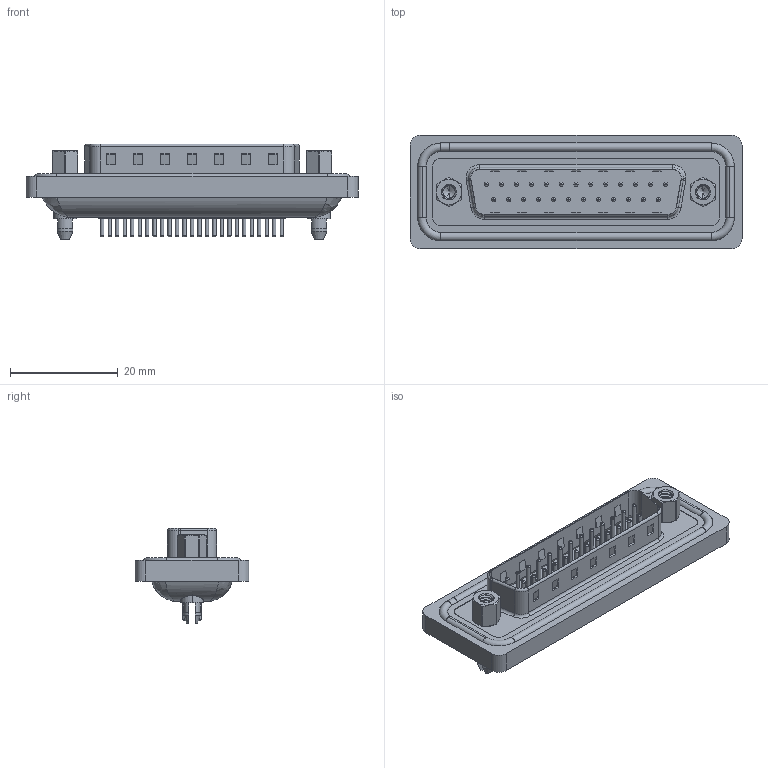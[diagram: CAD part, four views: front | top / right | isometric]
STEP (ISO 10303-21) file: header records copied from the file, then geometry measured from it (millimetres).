
FILE_DESCRIPTION (( 'STEP AP203' ), '1' );
FILE_NAME ('627-W25-220-013.STEP', '2021-04-05T19:34:12', ( '' ), ( '' ), 'SwSTEP 2.0', 'SolidWorks 2020', '' );
FILE_SCHEMA (( 'CONFIG_CONTROL_DESIGN' ));
Length unit declared in the file: millimetre
Products named in the file (8): 627W Contact Row 1_20; 627-W25-220-013; 627W Contact Row 2_20; 627W Shell Front_25 Contacts; 627W 4-40 Hex Standoff; 627W Waterproof Housing_25 Contacts BL; 627W Housing_25 Contacts; 627W 4-40 Threaded Boardlock
Assembly tree (32 placements, depth 2):
  627-W25-220-013
    627W Housing_25 Contacts
    627W Shell Front_25 Contacts
    627W Contact Row 1_20  x13
    627W Contact Row 2_20  x12
    627W Waterproof Housing_25 Contacts BL
    627W 4-40 Threaded Boardlock  x2
    627W 4-40 Hex Standoff  x2
Bounding box: 61.5 x 21.1 x 17.75 mm (x, y, z)
Volume: 7525.3 mm3; surface area: 11415.8 mm2
Topology: 33 solids, 33 shells, 1543 faces, 3488 edges, 2147 vertices
Faces by surface type: cylinder 652, torus 443, plane 394, cone 32, bspline 22
Entity records: 28412 total; most frequent: CARTESIAN_POINT 8299, DIRECTION 4084, ORIENTED_EDGE 3742, EDGE_CURVE 1871, AXIS2_PLACEMENT_3D 1607, VERTEX_POINT 1204, EDGE_LOOP 965, VECTOR 870
